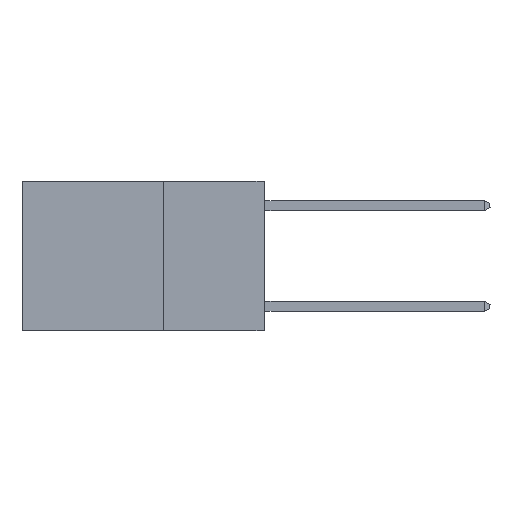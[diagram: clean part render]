
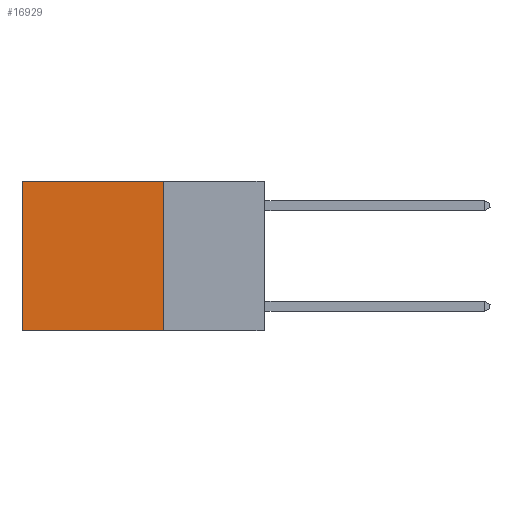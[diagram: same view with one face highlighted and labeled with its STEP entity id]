
A CAD part, left-side view. The second image highlights one B-rep face of the part: STEP entity #16929.
In plain terms, the highlighted planar face has unit normal (-1, 0, 0).
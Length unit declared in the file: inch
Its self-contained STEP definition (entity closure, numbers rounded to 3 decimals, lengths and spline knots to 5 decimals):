
#398 = DIRECTION ( 'NONE',  ( 0., 0., -1. ) ) ;
#540 = VERTEX_POINT ( 'NONE', #28701 ) ;
#2083 = FACE_OUTER_BOUND ( 'NONE', #10915, .T. ) ;
#2245 = CARTESIAN_POINT ( 'NONE',  ( 0.2625, 0.25, 0. ) ) ;
#3720 = CARTESIAN_POINT ( 'NONE',  ( 0.2625, 0.25, -0.37 ) ) ;
#3787 = VECTOR ( 'NONE', #398, 39.37008 ) ;
#3882 = VECTOR ( 'NONE', #7577, 39.37008 ) ;
#5782 = ORIENTED_EDGE ( 'NONE', *, *, #12320, .T. ) ;
#6547 = ORIENTED_EDGE ( 'NONE', *, *, #23429, .T. ) ;
#7577 = DIRECTION ( 'NONE',  ( 0., 1., 0. ) ) ;
#9085 = CARTESIAN_POINT ( 'NONE',  ( 0.2625, 0.25, 0. ) ) ;
#10915 = EDGE_LOOP ( 'NONE', ( #5782, #11570, #25972, #6547 ) ) ;
#11570 = ORIENTED_EDGE ( 'NONE', *, *, #23294, .F. ) ;
#11844 = EDGE_CURVE ( 'NONE', #17722, #540, #14037, .T. ) ;
#12320 = EDGE_CURVE ( 'NONE', #23769, #20262, #27043, .T. ) ;
#12914 = PLANE ( 'NONE',  #16531 ) ;
#13196 = CARTESIAN_POINT ( 'NONE',  ( 0.2625, 0.25, 0. ) ) ;
#14037 = LINE ( 'NONE', #9085, #21064 ) ;
#14959 = DIRECTION ( 'NONE',  ( 1., 0., 0. ) ) ;
#16499 = LINE ( 'NONE', #3720, #3882 ) ;
#16531 = AXIS2_PLACEMENT_3D ( 'NONE', #13196, #14959, #26092 ) ;
#16929 = ADVANCED_FACE ( 'NONE', ( #2083 ), #12914, .F. ) ;
#17722 = VERTEX_POINT ( 'NONE', #25705 ) ;
#18839 = VECTOR ( 'NONE', #26831, 39.37008 ) ;
#20262 = VERTEX_POINT ( 'NONE', #28765 ) ;
#20740 = CARTESIAN_POINT ( 'NONE',  ( 0.2625, 0.6, 0. ) ) ;
#21008 = CARTESIAN_POINT ( 'NONE',  ( 0.2625, 0.6, 0. ) ) ;
#21064 = VECTOR ( 'NONE', #25322, 39.37008 ) ;
#22301 = LINE ( 'NONE', #2245, #18839 ) ;
#23294 = EDGE_CURVE ( 'NONE', #540, #20262, #16499, .T. ) ;
#23429 = EDGE_CURVE ( 'NONE', #17722, #23769, #22301, .T. ) ;
#23769 = VERTEX_POINT ( 'NONE', #21008 ) ;
#25322 = DIRECTION ( 'NONE',  ( 0., 0., -1. ) ) ;
#25705 = CARTESIAN_POINT ( 'NONE',  ( 0.2625, 0.25, 0. ) ) ;
#25972 = ORIENTED_EDGE ( 'NONE', *, *, #11844, .F. ) ;
#26092 = DIRECTION ( 'NONE',  ( 0., 0., -1. ) ) ;
#26831 = DIRECTION ( 'NONE',  ( 0., 1., 0. ) ) ;
#27043 = LINE ( 'NONE', #20740, #3787 ) ;
#28701 = CARTESIAN_POINT ( 'NONE',  ( 0.2625, 0.25, -0.37 ) ) ;
#28765 = CARTESIAN_POINT ( 'NONE',  ( 0.2625, 0.6, -0.37 ) ) ;
